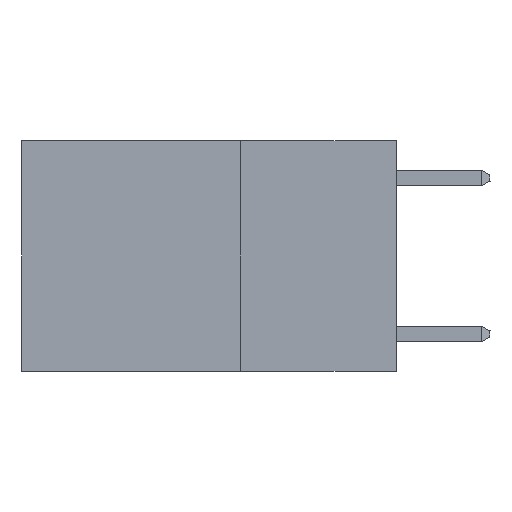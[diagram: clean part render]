
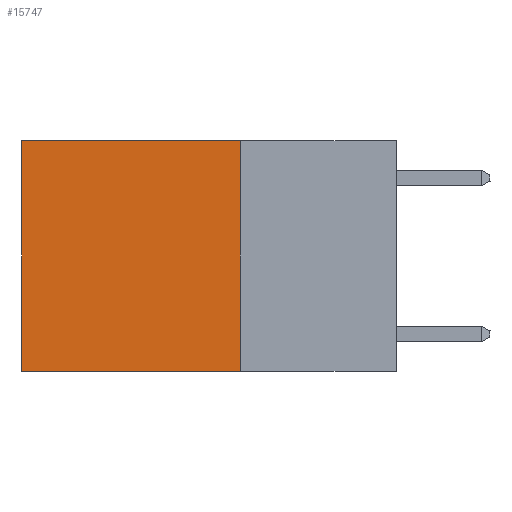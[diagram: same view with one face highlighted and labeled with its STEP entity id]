
A CAD part, left-side view. The second image highlights one B-rep face of the part: STEP entity #15747.
In plain terms, the highlighted planar face has unit normal (-1, 0, 0).
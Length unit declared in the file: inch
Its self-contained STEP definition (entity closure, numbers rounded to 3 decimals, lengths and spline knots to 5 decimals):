
#266 = ORIENTED_EDGE ( 'NONE', *, *, #22405, .F. ) ;
#918 = DIRECTION ( 'NONE',  ( 0., 1., 0. ) ) ;
#1586 = EDGE_CURVE ( 'NONE', #10029, #21830, #16116, .T. ) ;
#3092 = CARTESIAN_POINT ( 'NONE',  ( 0.2625, 0.25, -0.37 ) ) ;
#3548 = CARTESIAN_POINT ( 'NONE',  ( 0.2625, 0.6, 0. ) ) ;
#5988 = ORIENTED_EDGE ( 'NONE', *, *, #25432, .T. ) ;
#6867 = CARTESIAN_POINT ( 'NONE',  ( 0.2625, 0.25, 0. ) ) ;
#8423 = VERTEX_POINT ( 'NONE', #14597 ) ;
#9037 = VECTOR ( 'NONE', #918, 39.37008 ) ;
#9100 = VECTOR ( 'NONE', #18880, 39.37008 ) ;
#9673 = VERTEX_POINT ( 'NONE', #14119 ) ;
#10029 = VERTEX_POINT ( 'NONE', #3548 ) ;
#11009 = VECTOR ( 'NONE', #16667, 39.37008 ) ;
#11562 = EDGE_LOOP ( 'NONE', ( #16406, #20622, #266, #5988 ) ) ;
#11687 = LINE ( 'NONE', #3092, #23543 ) ;
#11821 = CARTESIAN_POINT ( 'NONE',  ( 0.2625, 0.6, 0. ) ) ;
#12933 = EDGE_CURVE ( 'NONE', #8423, #21830, #11687, .T. ) ;
#14119 = CARTESIAN_POINT ( 'NONE',  ( 0.2625, 0.25, 0. ) ) ;
#14597 = CARTESIAN_POINT ( 'NONE',  ( 0.2625, 0.25, -0.37 ) ) ;
#14738 = CARTESIAN_POINT ( 'NONE',  ( 0.2625, 0.6, -0.37 ) ) ;
#15747 = ADVANCED_FACE ( 'NONE', ( #23343 ), #23418, .F. ) ;
#16116 = LINE ( 'NONE', #11821, #9100 ) ;
#16350 = DIRECTION ( 'NONE',  ( 0., 0., -1. ) ) ;
#16406 = ORIENTED_EDGE ( 'NONE', *, *, #1586, .T. ) ;
#16667 = DIRECTION ( 'NONE',  ( 0., 0., -1. ) ) ;
#18028 = LINE ( 'NONE', #23835, #11009 ) ;
#18880 = DIRECTION ( 'NONE',  ( 0., 0., -1. ) ) ;
#19661 = DIRECTION ( 'NONE',  ( 0., 1., 0. ) ) ;
#20289 = AXIS2_PLACEMENT_3D ( 'NONE', #6867, #30499, #16350 ) ;
#20622 = ORIENTED_EDGE ( 'NONE', *, *, #12933, .F. ) ;
#21630 = LINE ( 'NONE', #22123, #9037 ) ;
#21830 = VERTEX_POINT ( 'NONE', #14738 ) ;
#22123 = CARTESIAN_POINT ( 'NONE',  ( 0.2625, 0.25, 0. ) ) ;
#22405 = EDGE_CURVE ( 'NONE', #9673, #8423, #18028, .T. ) ;
#23343 = FACE_OUTER_BOUND ( 'NONE', #11562, .T. ) ;
#23418 = PLANE ( 'NONE',  #20289 ) ;
#23543 = VECTOR ( 'NONE', #19661, 39.37008 ) ;
#23835 = CARTESIAN_POINT ( 'NONE',  ( 0.2625, 0.25, 0. ) ) ;
#25432 = EDGE_CURVE ( 'NONE', #9673, #10029, #21630, .T. ) ;
#30499 = DIRECTION ( 'NONE',  ( 1., 0., 0. ) ) ;
